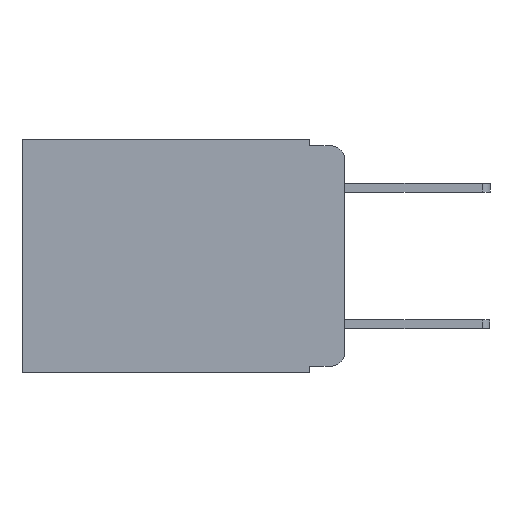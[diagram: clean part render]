
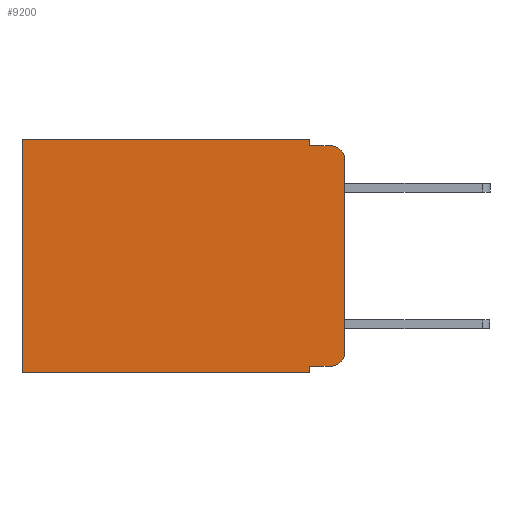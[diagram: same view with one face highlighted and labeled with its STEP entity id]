
A CAD part, left-side view. The second image highlights one B-rep face of the part: STEP entity #9200.
In plain terms, the highlighted planar face has unit normal (-1, 0, 0).
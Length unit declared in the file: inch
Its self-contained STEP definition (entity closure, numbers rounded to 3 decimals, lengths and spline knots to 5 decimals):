
#38 = LINE ( 'NONE', #4549, #22380 ) ;
#664 = CARTESIAN_POINT ( 'NONE',  ( 0.298, 0.051, -0.01 ) ) ;
#893 = DIRECTION ( 'NONE',  ( 0., 0., -1. ) ) ;
#966 = DIRECTION ( 'NONE',  ( 0., 0., -1. ) ) ;
#1169 = EDGE_LOOP ( 'NONE', ( #15834, #12845, #6683, #7168, #2076, #14356, #12761, #7973, #17327, #5049 ) ) ;
#2076 = ORIENTED_EDGE ( 'NONE', *, *, #15920, .T. ) ;
#3814 = LINE ( 'NONE', #19032, #11069 ) ;
#4395 = VERTEX_POINT ( 'NONE', #4687 ) ;
#4549 = CARTESIAN_POINT ( 'NONE',  ( 0.298, 0., 0. ) ) ;
#4687 = CARTESIAN_POINT ( 'NONE',  ( 0.298, 0.473, 0. ) ) ;
#4698 = VERTEX_POINT ( 'NONE', #20948 ) ;
#4746 = CARTESIAN_POINT ( 'NONE',  ( 0.298, 0.051, -0.333 ) ) ;
#4790 = CIRCLE ( 'NONE', #7738, 0.02 ) ;
#4834 = DIRECTION ( 'NONE',  ( 0., 1., 0. ) ) ;
#5049 = ORIENTED_EDGE ( 'NONE', *, *, #22015, .T. ) ;
#5097 = EDGE_CURVE ( 'NONE', #8876, #19249, #4790, .T. ) ;
#5107 = CARTESIAN_POINT ( 'NONE',  ( 0.298, 0.051, 0. ) ) ;
#5165 = EDGE_CURVE ( 'NONE', #13048, #18988, #21744, .T. ) ;
#5360 = CARTESIAN_POINT ( 'NONE',  ( 0.298, 0.02, -0.01 ) ) ;
#5611 = AXIS2_PLACEMENT_3D ( 'NONE', #6928, #19160, #8710 ) ;
#6683 = ORIENTED_EDGE ( 'NONE', *, *, #16201, .F. ) ;
#6928 = CARTESIAN_POINT ( 'NONE',  ( 0.298, 0.02, -0.313 ) ) ;
#7168 = ORIENTED_EDGE ( 'NONE', *, *, #19718, .F. ) ;
#7596 = EDGE_CURVE ( 'NONE', #4395, #21870, #21896, .T. ) ;
#7738 = AXIS2_PLACEMENT_3D ( 'NONE', #21981, #11645, #893 ) ;
#7973 = ORIENTED_EDGE ( 'NONE', *, *, #12363, .F. ) ;
#8461 = CARTESIAN_POINT ( 'NONE',  ( 0.298, 0., 0. ) ) ;
#8710 = DIRECTION ( 'NONE',  ( 0., 0., -1. ) ) ;
#8876 = VERTEX_POINT ( 'NONE', #21162 ) ;
#8912 = CARTESIAN_POINT ( 'NONE',  ( 0.298, 0.473, 0. ) ) ;
#8987 = DIRECTION ( 'NONE',  ( 0., 0., -1. ) ) ;
#9088 = LINE ( 'NONE', #664, #13814 ) ;
#9199 = DIRECTION ( 'NONE',  ( 0., -1., 0. ) ) ;
#9200 = ADVANCED_FACE ( 'NONE', ( #18780 ), #18927, .F. ) ;
#9831 = EDGE_CURVE ( 'NONE', #18414, #21870, #10303, .T. ) ;
#9930 = DIRECTION ( 'NONE',  ( 0., 0., -1. ) ) ;
#10227 = CARTESIAN_POINT ( 'NONE',  ( 0.298, 0.051, -0.333 ) ) ;
#10245 = DIRECTION ( 'NONE',  ( 0., 0., -1. ) ) ;
#10265 = VERTEX_POINT ( 'NONE', #19989 ) ;
#10303 = LINE ( 'NONE', #22257, #19012 ) ;
#10841 = CARTESIAN_POINT ( 'NONE',  ( 0.298, 0.051, 0. ) ) ;
#11069 = VECTOR ( 'NONE', #20733, 39.37008 ) ;
#11645 = DIRECTION ( 'NONE',  ( -1., 0., 0. ) ) ;
#11722 = CARTESIAN_POINT ( 'NONE',  ( 0.298, 0.051, 0. ) ) ;
#12303 = VECTOR ( 'NONE', #17783, 39.37008 ) ;
#12363 = EDGE_CURVE ( 'NONE', #13048, #18414, #16183, .T. ) ;
#12761 = ORIENTED_EDGE ( 'NONE', *, *, #9831, .F. ) ;
#12845 = ORIENTED_EDGE ( 'NONE', *, *, #5097, .T. ) ;
#12848 = LINE ( 'NONE', #10841, #12303 ) ;
#13048 = VERTEX_POINT ( 'NONE', #4746 ) ;
#13612 = CARTESIAN_POINT ( 'NONE',  ( 0.298, 0.473, -0.343 ) ) ;
#13814 = VECTOR ( 'NONE', #18358, 39.37008 ) ;
#14356 = ORIENTED_EDGE ( 'NONE', *, *, #7596, .T. ) ;
#15120 = VECTOR ( 'NONE', #966, 39.37008 ) ;
#15834 = ORIENTED_EDGE ( 'NONE', *, *, #20661, .F. ) ;
#15920 = EDGE_CURVE ( 'NONE', #20204, #4395, #3814, .T. ) ;
#16183 = LINE ( 'NONE', #11722, #15120 ) ;
#16201 = EDGE_CURVE ( 'NONE', #10265, #19249, #9088, .T. ) ;
#16651 = VECTOR ( 'NONE', #9199, 39.37008 ) ;
#17327 = ORIENTED_EDGE ( 'NONE', *, *, #5165, .T. ) ;
#17377 = VECTOR ( 'NONE', #8987, 39.37008 ) ;
#17783 = DIRECTION ( 'NONE',  ( 0., 0., -1. ) ) ;
#18358 = DIRECTION ( 'NONE',  ( 0., -1., 0. ) ) ;
#18414 = VERTEX_POINT ( 'NONE', #22352 ) ;
#18780 = FACE_OUTER_BOUND ( 'NONE', #1169, .T. ) ;
#18927 = PLANE ( 'NONE',  #20776 ) ;
#18988 = VERTEX_POINT ( 'NONE', #20368 ) ;
#19012 = VECTOR ( 'NONE', #4834, 39.37008 ) ;
#19032 = CARTESIAN_POINT ( 'NONE',  ( 0.298, 0., 0. ) ) ;
#19160 = DIRECTION ( 'NONE',  ( -1., 0., 0. ) ) ;
#19249 = VERTEX_POINT ( 'NONE', #5360 ) ;
#19718 = EDGE_CURVE ( 'NONE', #20204, #10265, #12848, .T. ) ;
#19989 = CARTESIAN_POINT ( 'NONE',  ( 0.298, 0.051, -0.01 ) ) ;
#20204 = VERTEX_POINT ( 'NONE', #5107 ) ;
#20368 = CARTESIAN_POINT ( 'NONE',  ( 0.298, 0.02, -0.333 ) ) ;
#20625 = DIRECTION ( 'NONE',  ( 1., 0., 0. ) ) ;
#20661 = EDGE_CURVE ( 'NONE', #8876, #4698, #38, .T. ) ;
#20733 = DIRECTION ( 'NONE',  ( 0., 1., 0. ) ) ;
#20776 = AXIS2_PLACEMENT_3D ( 'NONE', #8461, #20625, #10245 ) ;
#20948 = CARTESIAN_POINT ( 'NONE',  ( 0.298, 0., -0.313 ) ) ;
#21162 = CARTESIAN_POINT ( 'NONE',  ( 0.298, 0., -0.03 ) ) ;
#21744 = LINE ( 'NONE', #10227, #16651 ) ;
#21870 = VERTEX_POINT ( 'NONE', #13612 ) ;
#21896 = LINE ( 'NONE', #8912, #17377 ) ;
#21981 = CARTESIAN_POINT ( 'NONE',  ( 0.298, 0.02, -0.03 ) ) ;
#22015 = EDGE_CURVE ( 'NONE', #18988, #4698, #22321, .T. ) ;
#22257 = CARTESIAN_POINT ( 'NONE',  ( 0.298, 0., -0.343 ) ) ;
#22321 = CIRCLE ( 'NONE', #5611, 0.02 ) ;
#22352 = CARTESIAN_POINT ( 'NONE',  ( 0.298, 0.051, -0.343 ) ) ;
#22380 = VECTOR ( 'NONE', #9930, 39.37008 ) ;
